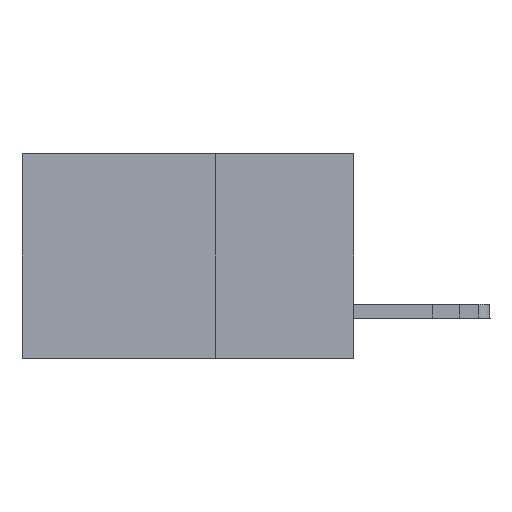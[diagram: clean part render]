
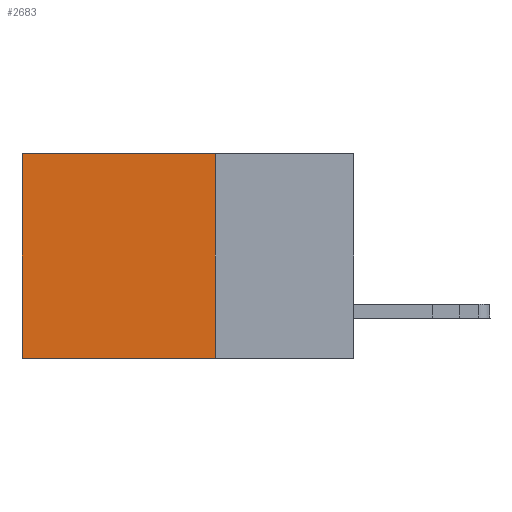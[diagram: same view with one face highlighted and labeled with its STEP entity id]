
A CAD part, left-side view. The second image highlights one B-rep face of the part: STEP entity #2683.
In plain terms, the highlighted planar face has unit normal (-1, 0, 0).
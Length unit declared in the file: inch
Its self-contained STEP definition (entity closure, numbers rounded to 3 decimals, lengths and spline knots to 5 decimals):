
#373 = ORIENTED_EDGE ( 'NONE', *, *, #12812, .T. ) ;
#1239 = EDGE_CURVE ( 'NONE', #14453, #15381, #12877, .T. ) ;
#1942 = CARTESIAN_POINT ( 'NONE',  ( 0.2875, 0.25, -0.37 ) ) ;
#2683 = ADVANCED_FACE ( 'NONE', ( #14581 ), #18103, .F. ) ;
#3621 = DIRECTION ( 'NONE',  ( 0., 1., 0. ) ) ;
#4326 = VECTOR ( 'NONE', #12690, 39.37008 ) ;
#5255 = DIRECTION ( 'NONE',  ( 0., 0., -1. ) ) ;
#7197 = CARTESIAN_POINT ( 'NONE',  ( 0.2875, 0.25, 0. ) ) ;
#8418 = VECTOR ( 'NONE', #16862, 39.37008 ) ;
#9059 = VERTEX_POINT ( 'NONE', #17381 ) ;
#9913 = EDGE_CURVE ( 'NONE', #9059, #18694, #16633, .T. ) ;
#11880 = EDGE_LOOP ( 'NONE', ( #373, #13817, #14383, #19234 ) ) ;
#11917 = EDGE_CURVE ( 'NONE', #14453, #9059, #17501, .T. ) ;
#12690 = DIRECTION ( 'NONE',  ( 0., 0., -1. ) ) ;
#12812 = EDGE_CURVE ( 'NONE', #15381, #18694, #12989, .T. ) ;
#12877 = LINE ( 'NONE', #19571, #20873 ) ;
#12989 = LINE ( 'NONE', #20578, #4326 ) ;
#13356 = CARTESIAN_POINT ( 'NONE',  ( 0.2875, 0.25, 0. ) ) ;
#13817 = ORIENTED_EDGE ( 'NONE', *, *, #9913, .F. ) ;
#14383 = ORIENTED_EDGE ( 'NONE', *, *, #11917, .F. ) ;
#14453 = VERTEX_POINT ( 'NONE', #19300 ) ;
#14581 = FACE_OUTER_BOUND ( 'NONE', #11880, .T. ) ;
#14968 = DIRECTION ( 'NONE',  ( 1., 0., 0. ) ) ;
#15381 = VERTEX_POINT ( 'NONE', #18708 ) ;
#16605 = DIRECTION ( 'NONE',  ( 0., 1., 0. ) ) ;
#16633 = LINE ( 'NONE', #1942, #19868 ) ;
#16862 = DIRECTION ( 'NONE',  ( 0., 0., -1. ) ) ;
#17381 = CARTESIAN_POINT ( 'NONE',  ( 0.2875, 0.25, -0.37 ) ) ;
#17501 = LINE ( 'NONE', #7197, #8418 ) ;
#18103 = PLANE ( 'NONE',  #19654 ) ;
#18694 = VERTEX_POINT ( 'NONE', #20871 ) ;
#18708 = CARTESIAN_POINT ( 'NONE',  ( 0.2875, 0.6, 0. ) ) ;
#19234 = ORIENTED_EDGE ( 'NONE', *, *, #1239, .T. ) ;
#19300 = CARTESIAN_POINT ( 'NONE',  ( 0.2875, 0.25, 0. ) ) ;
#19571 = CARTESIAN_POINT ( 'NONE',  ( 0.2875, 0.25, 0. ) ) ;
#19654 = AXIS2_PLACEMENT_3D ( 'NONE', #13356, #14968, #5255 ) ;
#19868 = VECTOR ( 'NONE', #3621, 39.37008 ) ;
#20578 = CARTESIAN_POINT ( 'NONE',  ( 0.2875, 0.6, 0. ) ) ;
#20871 = CARTESIAN_POINT ( 'NONE',  ( 0.2875, 0.6, -0.37 ) ) ;
#20873 = VECTOR ( 'NONE', #16605, 39.37008 ) ;
